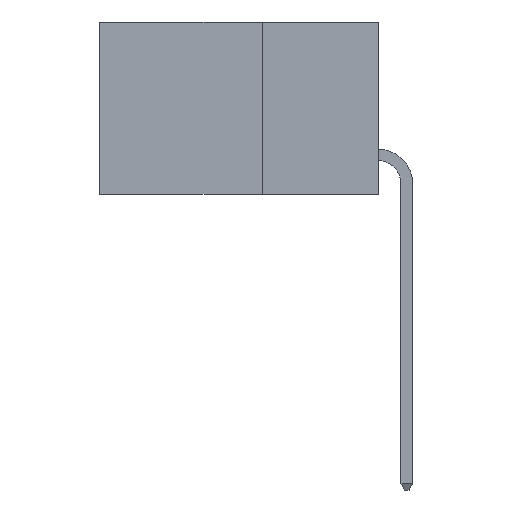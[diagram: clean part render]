
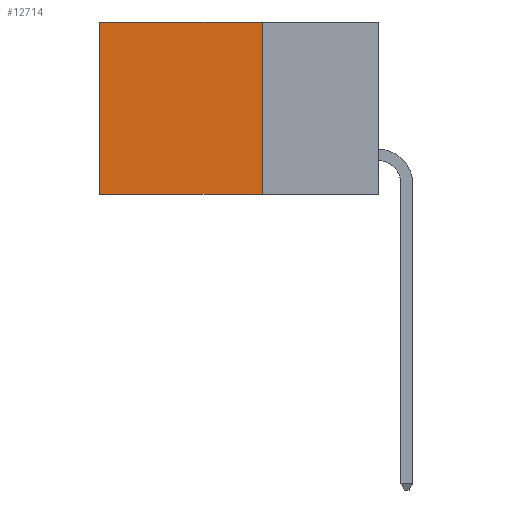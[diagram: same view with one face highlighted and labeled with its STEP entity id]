
A CAD part, left-side view. The second image highlights one B-rep face of the part: STEP entity #12714.
In plain terms, the highlighted planar face has unit normal (-1, 0, 0).
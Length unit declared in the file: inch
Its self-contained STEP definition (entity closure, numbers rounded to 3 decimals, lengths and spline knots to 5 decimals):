
#1554 = CARTESIAN_POINT ( 'NONE',  ( 0.2615, 0.6, 0. ) ) ;
#2101 = LINE ( 'NONE', #14677, #14641 ) ;
#2222 = DIRECTION ( 'NONE',  ( 0., 0., -1. ) ) ;
#2408 = ORIENTED_EDGE ( 'NONE', *, *, #9947, .F. ) ;
#2693 = FACE_OUTER_BOUND ( 'NONE', #17778, .T. ) ;
#2884 = ORIENTED_EDGE ( 'NONE', *, *, #3127, .F. ) ;
#2993 = AXIS2_PLACEMENT_3D ( 'NONE', #7745, #18221, #9246 ) ;
#3127 = EDGE_CURVE ( 'NONE', #18890, #10176, #12165, .T. ) ;
#3203 = PLANE ( 'NONE',  #2993 ) ;
#7038 = VERTEX_POINT ( 'NONE', #1554 ) ;
#7126 = VECTOR ( 'NONE', #11897, 39.37008 ) ;
#7307 = VERTEX_POINT ( 'NONE', #11442 ) ;
#7745 = CARTESIAN_POINT ( 'NONE',  ( 0.2615, 0.25, -0.37 ) ) ;
#8292 = CARTESIAN_POINT ( 'NONE',  ( 0.2615, 0.6, -0.37 ) ) ;
#9246 = DIRECTION ( 'NONE',  ( 0., 0., -1. ) ) ;
#9618 = VECTOR ( 'NONE', #2222, 39.37008 ) ;
#9947 = EDGE_CURVE ( 'NONE', #10176, #7307, #2101, .T. ) ;
#10096 = DIRECTION ( 'NONE',  ( 0., 1., 0. ) ) ;
#10176 = VERTEX_POINT ( 'NONE', #15203 ) ;
#10417 = EDGE_CURVE ( 'NONE', #7038, #7307, #13676, .T. ) ;
#10836 = DIRECTION ( 'NONE',  ( 0., 0., -1. ) ) ;
#10875 = CARTESIAN_POINT ( 'NONE',  ( 0.2615, 0.25, -0.37 ) ) ;
#11138 = LINE ( 'NONE', #16422, #7126 ) ;
#11367 = CARTESIAN_POINT ( 'NONE',  ( 0.2615, 0.25, 0. ) ) ;
#11442 = CARTESIAN_POINT ( 'NONE',  ( 0.2615, 0.6, -0.37 ) ) ;
#11897 = DIRECTION ( 'NONE',  ( 0., 1., 0. ) ) ;
#12165 = LINE ( 'NONE', #10875, #15711 ) ;
#12714 = ADVANCED_FACE ( 'NONE', ( #2693 ), #3203, .F. ) ;
#13676 = LINE ( 'NONE', #8292, #9618 ) ;
#14641 = VECTOR ( 'NONE', #10096, 39.37008 ) ;
#14677 = CARTESIAN_POINT ( 'NONE',  ( 0.2615, 0.25, -0.37 ) ) ;
#15203 = CARTESIAN_POINT ( 'NONE',  ( 0.2615, 0.25, -0.37 ) ) ;
#15505 = ORIENTED_EDGE ( 'NONE', *, *, #16869, .T. ) ;
#15711 = VECTOR ( 'NONE', #10836, 39.37008 ) ;
#16422 = CARTESIAN_POINT ( 'NONE',  ( 0.2615, 0.25, 0. ) ) ;
#16869 = EDGE_CURVE ( 'NONE', #18890, #7038, #11138, .T. ) ;
#17778 = EDGE_LOOP ( 'NONE', ( #19491, #2408, #2884, #15505 ) ) ;
#18221 = DIRECTION ( 'NONE',  ( 1., 0., 0. ) ) ;
#18890 = VERTEX_POINT ( 'NONE', #11367 ) ;
#19491 = ORIENTED_EDGE ( 'NONE', *, *, #10417, .T. ) ;
